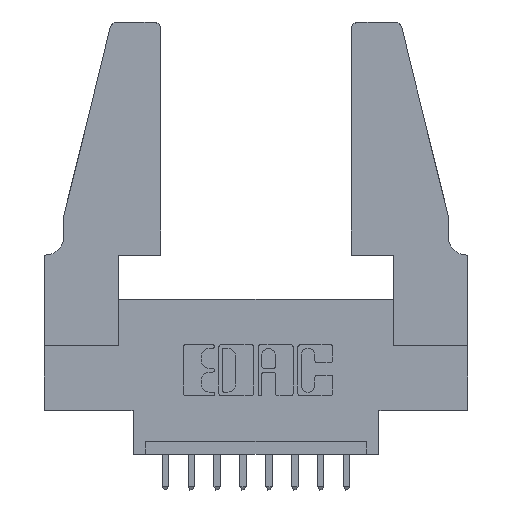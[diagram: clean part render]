
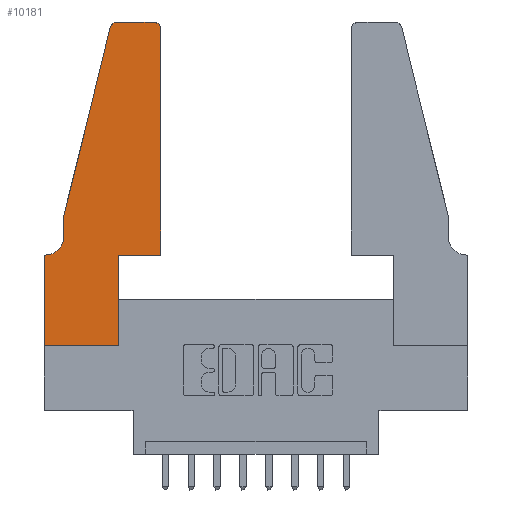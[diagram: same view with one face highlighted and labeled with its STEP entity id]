
A CAD part, top view. The second image highlights one B-rep face of the part: STEP entity #10181.
In plain terms, the highlighted planar face has unit normal (0, 0, 1).
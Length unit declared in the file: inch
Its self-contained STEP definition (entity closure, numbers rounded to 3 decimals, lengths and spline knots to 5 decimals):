
#27 = DIRECTION ( 'NONE',  ( 0., -1., 0. ) ) ;
#121 = CARTESIAN_POINT ( 'NONE',  ( 0.2865, 0., 0.37 ) ) ;
#502 = VECTOR ( 'NONE', #10301, 39.37008 ) ;
#674 = CARTESIAN_POINT ( 'NONE',  ( 0., 0.35, 0.37 ) ) ;
#775 = VERTEX_POINT ( 'NONE', #11113 ) ;
#809 = CARTESIAN_POINT ( 'NONE',  ( 0.0755, 0.5, 0.37 ) ) ;
#962 = ORIENTED_EDGE ( 'NONE', *, *, #1799, .T. ) ;
#1064 = VECTOR ( 'NONE', #2355, 39.37008 ) ;
#1070 = CARTESIAN_POINT ( 'NONE',  ( 0.0755, 0.5, 0.37 ) ) ;
#1199 = AXIS2_PLACEMENT_3D ( 'NONE', #674, #7629, #2602 ) ;
#1453 = EDGE_CURVE ( 'NONE', #9608, #9117, #10293, .T. ) ;
#1479 = DIRECTION ( 'NONE',  ( 1., 0., 0. ) ) ;
#1560 = CIRCLE ( 'NONE', #2356, 0.07 ) ;
#1799 = EDGE_CURVE ( 'NONE', #8772, #775, #10745, .T. ) ;
#2226 = CARTESIAN_POINT ( 'NONE',  ( 0.4505, 0.35, 0.37 ) ) ;
#2355 = DIRECTION ( 'NONE',  ( 0., -1., 0. ) ) ;
#2356 = AXIS2_PLACEMENT_3D ( 'NONE', #12430, #7338, #8428 ) ;
#2602 = DIRECTION ( 'NONE',  ( 1., 0., 0. ) ) ;
#2795 = VERTEX_POINT ( 'NONE', #12547 ) ;
#2873 = VECTOR ( 'NONE', #8382, 39.37008 ) ;
#3430 = DIRECTION ( 'NONE',  ( -1., 0., 0. ) ) ;
#3576 = LINE ( 'NONE', #9469, #502 ) ;
#3687 = CARTESIAN_POINT ( 'NONE',  ( 0.0055, 0.35, 0.37 ) ) ;
#3982 = DIRECTION ( 'NONE',  ( 1., 0., 0. ) ) ;
#4090 = EDGE_CURVE ( 'NONE', #10129, #12281, #9586, .T. ) ;
#4195 = ORIENTED_EDGE ( 'NONE', *, *, #11217, .T. ) ;
#4335 = EDGE_CURVE ( 'NONE', #9384, #8772, #9601, .T. ) ;
#4413 = VERTEX_POINT ( 'NONE', #809 ) ;
#4513 = PLANE ( 'NONE',  #1199 ) ;
#4535 = VERTEX_POINT ( 'NONE', #11039 ) ;
#4723 = CARTESIAN_POINT ( 'NONE',  ( 0., 0.35, 0.37 ) ) ;
#5029 = ORIENTED_EDGE ( 'NONE', *, *, #9866, .T. ) ;
#5031 = AXIS2_PLACEMENT_3D ( 'NONE', #7623, #12618, #1479 ) ;
#5367 = DIRECTION ( 'NONE',  ( 0., 1., 0. ) ) ;
#5642 = CARTESIAN_POINT ( 'NONE',  ( 0.2865, 0.35, 0.37 ) ) ;
#6020 = DIRECTION ( 'NONE',  ( -0.239, -0.971, 0. ) ) ;
#6049 = LINE ( 'NONE', #8347, #1064 ) ;
#6147 = FACE_OUTER_BOUND ( 'NONE', #10250, .T. ) ;
#6699 = CARTESIAN_POINT ( 'NONE',  ( 0.4205, 1.25, 0.37 ) ) ;
#6941 = DIRECTION ( 'NONE',  ( 0., 0., 1. ) ) ;
#7025 = VERTEX_POINT ( 'NONE', #9827 ) ;
#7085 = DIRECTION ( 'NONE',  ( -1., 0., 0. ) ) ;
#7291 = ORIENTED_EDGE ( 'NONE', *, *, #7782, .T. ) ;
#7338 = DIRECTION ( 'NONE',  ( 0., 0., -1. ) ) ;
#7347 = ORIENTED_EDGE ( 'NONE', *, *, #4335, .T. ) ;
#7418 = CARTESIAN_POINT ( 'NONE',  ( 0.4505, 1.22, 0.37 ) ) ;
#7623 = CARTESIAN_POINT ( 'NONE',  ( 0.284, 1.22, 0.37 ) ) ;
#7629 = DIRECTION ( 'NONE',  ( 0., 0., 1. ) ) ;
#7678 = LINE ( 'NONE', #1070, #11443 ) ;
#7782 = EDGE_CURVE ( 'NONE', #9117, #7025, #6049, .T. ) ;
#7845 = EDGE_CURVE ( 'NONE', #4535, #4413, #12753, .T. ) ;
#7948 = DIRECTION ( 'NONE',  ( 1., 0., 0. ) ) ;
#7992 = ORIENTED_EDGE ( 'NONE', *, *, #10020, .T. ) ;
#8034 = ORIENTED_EDGE ( 'NONE', *, *, #1453, .T. ) ;
#8320 = ORIENTED_EDGE ( 'NONE', *, *, #11395, .T. ) ;
#8347 = CARTESIAN_POINT ( 'NONE',  ( 0., 0., 0.37 ) ) ;
#8382 = DIRECTION ( 'NONE',  ( 0., 1., 0. ) ) ;
#8428 = DIRECTION ( 'NONE',  ( -1., 0., 0. ) ) ;
#8772 = VERTEX_POINT ( 'NONE', #6699 ) ;
#8790 = LINE ( 'NONE', #2226, #11608 ) ;
#9075 = CIRCLE ( 'NONE', #5031, 0.03 ) ;
#9117 = VERTEX_POINT ( 'NONE', #4723 ) ;
#9265 = ORIENTED_EDGE ( 'NONE', *, *, #12809, .T. ) ;
#9377 = CARTESIAN_POINT ( 'NONE',  ( 0.4205, 1.22, 0.37 ) ) ;
#9384 = VERTEX_POINT ( 'NONE', #7418 ) ;
#9469 = CARTESIAN_POINT ( 'NONE',  ( 0., 0., 0.37 ) ) ;
#9586 = LINE ( 'NONE', #10516, #2873 ) ;
#9601 = CIRCLE ( 'NONE', #11456, 0.03 ) ;
#9608 = VERTEX_POINT ( 'NONE', #3687 ) ;
#9827 = CARTESIAN_POINT ( 'NONE',  ( 0., 0., 0.37 ) ) ;
#9866 = EDGE_CURVE ( 'NONE', #2795, #9384, #8790, .T. ) ;
#9876 = CARTESIAN_POINT ( 'NONE',  ( 0.0755, 0.42, 0.37 ) ) ;
#10020 = EDGE_CURVE ( 'NONE', #4413, #12136, #7678, .T. ) ;
#10035 = CARTESIAN_POINT ( 'NONE',  ( 0.0755, 0.35, 0.37 ) ) ;
#10129 = VERTEX_POINT ( 'NONE', #121 ) ;
#10181 = ADVANCED_FACE ( 'NONE', ( #6147 ), #4513, .T. ) ;
#10250 = EDGE_LOOP ( 'NONE', ( #962, #8320, #11689, #7992, #4195, #8034, #7291, #12504, #11088, #9265, #5029, #7347 ) ) ;
#10270 = CARTESIAN_POINT ( 'NONE',  ( 0.2605, 1.25, 0.37 ) ) ;
#10293 = LINE ( 'NONE', #10035, #11895 ) ;
#10301 = DIRECTION ( 'NONE',  ( 1., 0., 0. ) ) ;
#10516 = CARTESIAN_POINT ( 'NONE',  ( 0.2865, 0.35, 0.37 ) ) ;
#10589 = VECTOR ( 'NONE', #3430, 39.37008 ) ;
#10745 = LINE ( 'NONE', #10270, #10589 ) ;
#10849 = EDGE_CURVE ( 'NONE', #7025, #10129, #3576, .T. ) ;
#11032 = VECTOR ( 'NONE', #6020, 39.37008 ) ;
#11039 = CARTESIAN_POINT ( 'NONE',  ( 0.25487, 1.22718, 0.37 ) ) ;
#11053 = LINE ( 'NONE', #12325, #12927 ) ;
#11088 = ORIENTED_EDGE ( 'NONE', *, *, #4090, .T. ) ;
#11113 = CARTESIAN_POINT ( 'NONE',  ( 0.284, 1.25, 0.37 ) ) ;
#11217 = EDGE_CURVE ( 'NONE', #12136, #9608, #1560, .T. ) ;
#11395 = EDGE_CURVE ( 'NONE', #775, #4535, #9075, .T. ) ;
#11443 = VECTOR ( 'NONE', #27, 39.37008 ) ;
#11456 = AXIS2_PLACEMENT_3D ( 'NONE', #9377, #6941, #7948 ) ;
#11608 = VECTOR ( 'NONE', #5367, 39.37008 ) ;
#11689 = ORIENTED_EDGE ( 'NONE', *, *, #7845, .T. ) ;
#11862 = CARTESIAN_POINT ( 'NONE',  ( 0.0755, 0.5, 0.37 ) ) ;
#11895 = VECTOR ( 'NONE', #7085, 39.37008 ) ;
#12136 = VERTEX_POINT ( 'NONE', #9876 ) ;
#12281 = VERTEX_POINT ( 'NONE', #5642 ) ;
#12325 = CARTESIAN_POINT ( 'NONE',  ( 0.4505, 0.35, 0.37 ) ) ;
#12430 = CARTESIAN_POINT ( 'NONE',  ( 0.0055, 0.42, 0.37 ) ) ;
#12504 = ORIENTED_EDGE ( 'NONE', *, *, #10849, .T. ) ;
#12547 = CARTESIAN_POINT ( 'NONE',  ( 0.4505, 0.35, 0.37 ) ) ;
#12618 = DIRECTION ( 'NONE',  ( 0., 0., 1. ) ) ;
#12753 = LINE ( 'NONE', #11862, #11032 ) ;
#12809 = EDGE_CURVE ( 'NONE', #12281, #2795, #11053, .T. ) ;
#12927 = VECTOR ( 'NONE', #3982, 39.37008 ) ;
